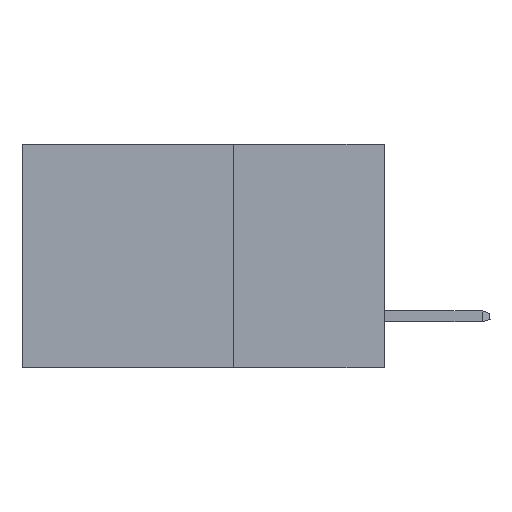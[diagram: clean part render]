
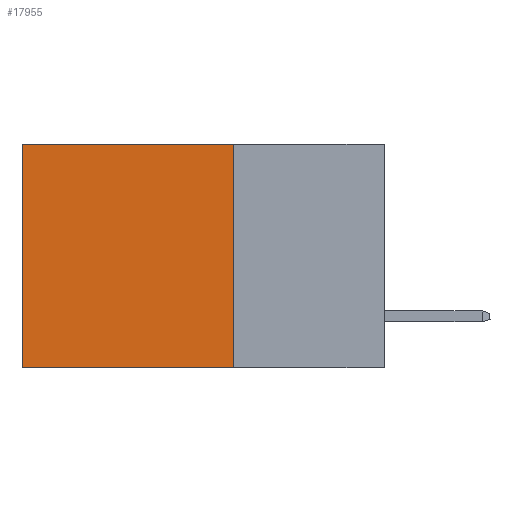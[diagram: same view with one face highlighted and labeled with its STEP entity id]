
A CAD part, left-side view. The second image highlights one B-rep face of the part: STEP entity #17955.
In plain terms, the highlighted planar face has unit normal (-1, 0, 0).
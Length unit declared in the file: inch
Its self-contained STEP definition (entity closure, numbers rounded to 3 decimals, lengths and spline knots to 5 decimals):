
#202 = DIRECTION ( 'NONE',  ( 0., 1., 0. ) ) ;
#366 = ORIENTED_EDGE ( 'NONE', *, *, #511, .F. ) ;
#511 = EDGE_CURVE ( 'NONE', #16984, #16252, #1470, .T. ) ;
#1470 = LINE ( 'NONE', #6127, #16150 ) ;
#2228 = CARTESIAN_POINT ( 'NONE',  ( 0.298, 0.6, 0. ) ) ;
#2537 = DIRECTION ( 'NONE',  ( 0., 0., -1. ) ) ;
#2933 = DIRECTION ( 'NONE',  ( 0., 0., -1. ) ) ;
#3218 = EDGE_CURVE ( 'NONE', #17881, #6629, #16615, .T. ) ;
#3860 = ORIENTED_EDGE ( 'NONE', *, *, #3218, .T. ) ;
#3940 = DIRECTION ( 'NONE',  ( 0., 1., 0. ) ) ;
#6096 = CARTESIAN_POINT ( 'NONE',  ( 0.298, 0.25, 0. ) ) ;
#6127 = CARTESIAN_POINT ( 'NONE',  ( 0.298, 0.25, 0. ) ) ;
#6465 = AXIS2_PLACEMENT_3D ( 'NONE', #6096, #15002, #2933 ) ;
#6629 = VERTEX_POINT ( 'NONE', #12312 ) ;
#6964 = FACE_OUTER_BOUND ( 'NONE', #18567, .T. ) ;
#7901 = EDGE_CURVE ( 'NONE', #16252, #6629, #10566, .T. ) ;
#8062 = EDGE_CURVE ( 'NONE', #16984, #17881, #13676, .T. ) ;
#9059 = ORIENTED_EDGE ( 'NONE', *, *, #7901, .F. ) ;
#9127 = VECTOR ( 'NONE', #202, 39.37008 ) ;
#9594 = VECTOR ( 'NONE', #3940, 39.37008 ) ;
#10566 = LINE ( 'NONE', #16832, #9127 ) ;
#11376 = CARTESIAN_POINT ( 'NONE',  ( 0.298, 0.25, 0. ) ) ;
#11466 = ORIENTED_EDGE ( 'NONE', *, *, #8062, .T. ) ;
#11713 = CARTESIAN_POINT ( 'NONE',  ( 0.298, 0.25, 0. ) ) ;
#12246 = DIRECTION ( 'NONE',  ( 0., 0., -1. ) ) ;
#12312 = CARTESIAN_POINT ( 'NONE',  ( 0.298, 0.6, -0.37 ) ) ;
#13676 = LINE ( 'NONE', #11376, #9594 ) ;
#14723 = VECTOR ( 'NONE', #2537, 39.37008 ) ;
#15002 = DIRECTION ( 'NONE',  ( 1., 0., 0. ) ) ;
#16150 = VECTOR ( 'NONE', #12246, 39.37008 ) ;
#16252 = VERTEX_POINT ( 'NONE', #16875 ) ;
#16615 = LINE ( 'NONE', #2228, #14723 ) ;
#16832 = CARTESIAN_POINT ( 'NONE',  ( 0.298, 0.25, -0.37 ) ) ;
#16875 = CARTESIAN_POINT ( 'NONE',  ( 0.298, 0.25, -0.37 ) ) ;
#16984 = VERTEX_POINT ( 'NONE', #11713 ) ;
#17881 = VERTEX_POINT ( 'NONE', #18040 ) ;
#17955 = ADVANCED_FACE ( 'NONE', ( #6964 ), #18235, .F. ) ;
#18040 = CARTESIAN_POINT ( 'NONE',  ( 0.298, 0.6, 0. ) ) ;
#18235 = PLANE ( 'NONE',  #6465 ) ;
#18567 = EDGE_LOOP ( 'NONE', ( #3860, #9059, #366, #11466 ) ) ;
